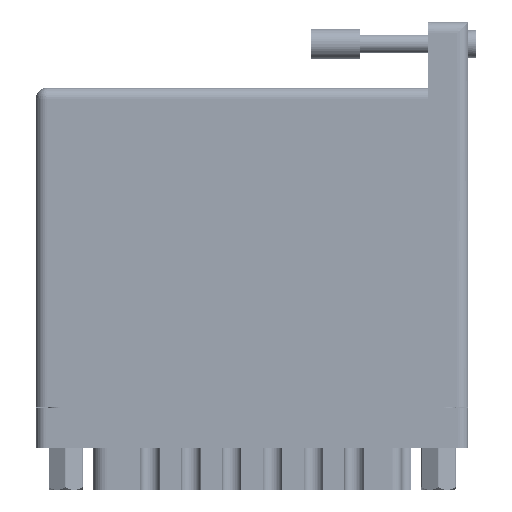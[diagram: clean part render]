
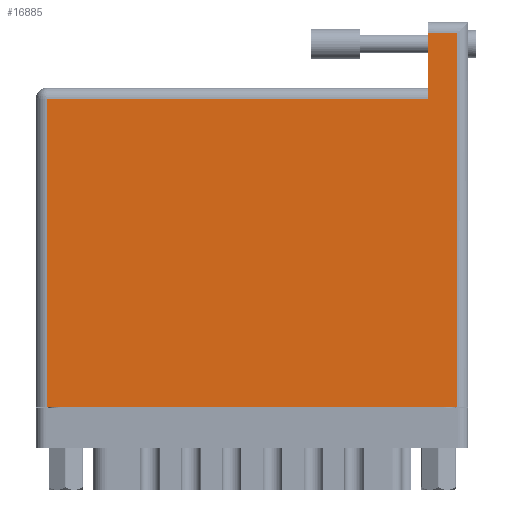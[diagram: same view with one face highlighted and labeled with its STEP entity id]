
A CAD part, front view. The second image highlights one B-rep face of the part: STEP entity #16885.
In plain terms, the highlighted face is planar.
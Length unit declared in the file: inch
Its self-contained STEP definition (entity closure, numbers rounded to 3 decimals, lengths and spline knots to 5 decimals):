
#286 = CARTESIAN_POINT ( 'NONE',  ( 0.07, 0., 0. ) ) ;
#1332 = EDGE_CURVE ( 'NONE', #91384, #90528, #59415, .T. ) ;
#1984 = CARTESIAN_POINT ( 'NONE',  ( 0.07, 1.96, 0. ) ) ;
#2068 = DIRECTION ( 'NONE',  ( -1., 0., 0. ) ) ;
#2430 = PLANE ( 'NONE',  #56800 ) ;
#4802 = EDGE_CURVE ( 'NONE', #8341, #25975, #60356, .T. ) ;
#6092 = LINE ( 'NONE', #101619, #21404 ) ;
#8341 = VERTEX_POINT ( 'NONE', #1984 ) ;
#16434 = VERTEX_POINT ( 'NONE', #27826 ) ;
#16885 = ADVANCED_FACE ( 'NONE', ( #60848 ), #2430, .F. ) ;
#18226 = CARTESIAN_POINT ( 'NONE',  ( 0.07, 0., 0. ) ) ;
#21404 = VECTOR ( 'NONE', #27988, 39.37008 ) ;
#25682 = LINE ( 'NONE', #64877, #48685 ) ;
#25975 = VERTEX_POINT ( 'NONE', #18226 ) ;
#27826 = CARTESIAN_POINT ( 'NONE',  ( 2.499, 1.96, 0. ) ) ;
#27988 = DIRECTION ( 'NONE',  ( 1., 0., 0. ) ) ;
#28284 = VERTEX_POINT ( 'NONE', #88401 ) ;
#31366 = DIRECTION ( 'NONE',  ( 0., 1., 0. ) ) ;
#32790 = CARTESIAN_POINT ( 'NONE',  ( 2.685, 0., 0. ) ) ;
#41023 = LINE ( 'NONE', #100133, #92202 ) ;
#46940 = ORIENTED_EDGE ( 'NONE', *, *, #4802, .T. ) ;
#48685 = VECTOR ( 'NONE', #105329, 39.37008 ) ;
#50130 = ORIENTED_EDGE ( 'NONE', *, *, #77076, .T. ) ;
#50138 = VECTOR ( 'NONE', #97507, 39.37008 ) ;
#51304 = EDGE_CURVE ( 'NONE', #28284, #16434, #41023, .T. ) ;
#52359 = CARTESIAN_POINT ( 'NONE',  ( 0., 2.03, 0. ) ) ;
#54920 = CARTESIAN_POINT ( 'NONE',  ( 2.685, 2.45, 0. ) ) ;
#56800 = AXIS2_PLACEMENT_3D ( 'NONE', #52359, #68787, #2068 ) ;
#59019 = DIRECTION ( 'NONE',  ( -1., 0., 0. ) ) ;
#59415 = LINE ( 'NONE', #54920, #87574 ) ;
#60356 = LINE ( 'NONE', #286, #50138 ) ;
#60848 = FACE_OUTER_BOUND ( 'NONE', #74846, .T. ) ;
#63386 = VECTOR ( 'NONE', #59019, 39.37008 ) ;
#64877 = CARTESIAN_POINT ( 'NONE',  ( 0., 2.38, 0. ) ) ;
#68787 = DIRECTION ( 'NONE',  ( 0., 0., -1. ) ) ;
#69038 = EDGE_CURVE ( 'NONE', #16434, #8341, #86519, .T. ) ;
#72349 = ORIENTED_EDGE ( 'NONE', *, *, #51304, .T. ) ;
#74417 = CARTESIAN_POINT ( 'NONE',  ( 0., 1.96, 0. ) ) ;
#74846 = EDGE_LOOP ( 'NONE', ( #72349, #82532, #46940, #50130, #97138, #103605 ) ) ;
#77076 = EDGE_CURVE ( 'NONE', #25975, #91384, #6092, .T. ) ;
#82532 = ORIENTED_EDGE ( 'NONE', *, *, #69038, .T. ) ;
#86519 = LINE ( 'NONE', #74417, #63386 ) ;
#87574 = VECTOR ( 'NONE', #31366, 39.37008 ) ;
#88401 = CARTESIAN_POINT ( 'NONE',  ( 2.499, 2.38, 0. ) ) ;
#90266 = EDGE_CURVE ( 'NONE', #90528, #28284, #25682, .T. ) ;
#90528 = VERTEX_POINT ( 'NONE', #101207 ) ;
#91384 = VERTEX_POINT ( 'NONE', #32790 ) ;
#92202 = VECTOR ( 'NONE', #99788, 39.37008 ) ;
#97138 = ORIENTED_EDGE ( 'NONE', *, *, #1332, .T. ) ;
#97507 = DIRECTION ( 'NONE',  ( 0., -1., 0. ) ) ;
#99788 = DIRECTION ( 'NONE',  ( 0., -1., 0. ) ) ;
#100133 = CARTESIAN_POINT ( 'NONE',  ( 2.499, 2.45, 0. ) ) ;
#101207 = CARTESIAN_POINT ( 'NONE',  ( 2.685, 2.38, 0. ) ) ;
#101619 = CARTESIAN_POINT ( 'NONE',  ( 0., 0., 0. ) ) ;
#103605 = ORIENTED_EDGE ( 'NONE', *, *, #90266, .T. ) ;
#105329 = DIRECTION ( 'NONE',  ( -1., 0., 0. ) ) ;
